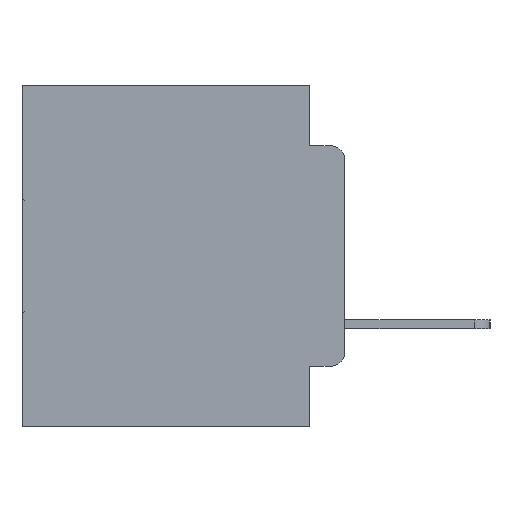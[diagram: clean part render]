
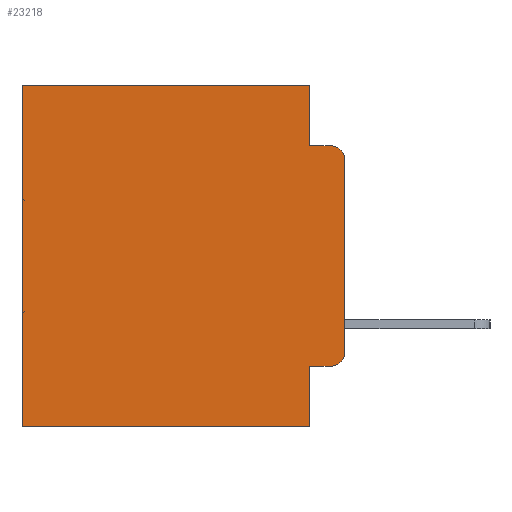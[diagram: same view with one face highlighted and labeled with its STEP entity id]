
A CAD part, left-side view. The second image highlights one B-rep face of the part: STEP entity #23218.
In plain terms, the highlighted planar face has unit normal (-1, 0, 0).
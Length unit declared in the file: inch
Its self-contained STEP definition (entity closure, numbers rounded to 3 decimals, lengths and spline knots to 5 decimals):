
#215 = DIRECTION ( 'NONE',  ( 0., 0., -1. ) ) ;
#223 = LINE ( 'NONE', #2752, #25096 ) ;
#811 = EDGE_CURVE ( 'NONE', #27575, #18160, #24040, .T. ) ;
#1923 = EDGE_CURVE ( 'NONE', #21573, #21307, #223, .T. ) ;
#2181 = CARTESIAN_POINT ( 'NONE',  ( 0.298, 0., 0. ) ) ;
#2608 = EDGE_CURVE ( 'NONE', #27176, #14300, #9049, .T. ) ;
#2657 = CARTESIAN_POINT ( 'NONE',  ( 0.298, 0., -0.5 ) ) ;
#2752 = CARTESIAN_POINT ( 'NONE',  ( 0.298, 0.051, -0.0885 ) ) ;
#2983 = CARTESIAN_POINT ( 'NONE',  ( 0.298, 0.02, -0.4115 ) ) ;
#3525 = EDGE_LOOP ( 'NONE', ( #14341, #7634, #15775, #22867, #12550, #25723, #14309, #5526, #22496, #13856 ) ) ;
#4274 = CARTESIAN_POINT ( 'NONE',  ( 0.298, 0.02, -0.3915 ) ) ;
#4275 = LINE ( 'NONE', #25701, #15556 ) ;
#4698 = DIRECTION ( 'NONE',  ( -1., 0., 0. ) ) ;
#5526 = ORIENTED_EDGE ( 'NONE', *, *, #7463, .F. ) ;
#6315 = VERTEX_POINT ( 'NONE', #19563 ) ;
#6690 = DIRECTION ( 'NONE',  ( 0., 0., -1. ) ) ;
#7463 = EDGE_CURVE ( 'NONE', #27575, #27176, #10236, .T. ) ;
#7634 = ORIENTED_EDGE ( 'NONE', *, *, #8484, .T. ) ;
#7880 = CIRCLE ( 'NONE', #20224, 0.02 ) ;
#8484 = EDGE_CURVE ( 'NONE', #24120, #21307, #11255, .T. ) ;
#9049 = LINE ( 'NONE', #2657, #14660 ) ;
#9115 = DIRECTION ( 'NONE',  ( 0., 0., -1. ) ) ;
#9828 = CARTESIAN_POINT ( 'NONE',  ( 0.298, 0., 0. ) ) ;
#9999 = DIRECTION ( 'NONE',  ( 0., 1., 0. ) ) ;
#10236 = LINE ( 'NONE', #17215, #22881 ) ;
#10637 = VECTOR ( 'NONE', #28673, 39.37008 ) ;
#10702 = CARTESIAN_POINT ( 'NONE',  ( 0.298, 0., -0.1085 ) ) ;
#10851 = VECTOR ( 'NONE', #9999, 39.37008 ) ;
#11255 = CIRCLE ( 'NONE', #20535, 0.02 ) ;
#11478 = DIRECTION ( 'NONE',  ( 0., 0., -1. ) ) ;
#11507 = CARTESIAN_POINT ( 'NONE',  ( 0.298, 0.473, 0. ) ) ;
#12235 = DIRECTION ( 'NONE',  ( 0., 0., -1. ) ) ;
#12550 = ORIENTED_EDGE ( 'NONE', *, *, #15513, .T. ) ;
#13628 = CARTESIAN_POINT ( 'NONE',  ( 0.298, 0.02, -0.0885 ) ) ;
#13856 = ORIENTED_EDGE ( 'NONE', *, *, #22452, .T. ) ;
#14300 = VERTEX_POINT ( 'NONE', #23668 ) ;
#14309 = ORIENTED_EDGE ( 'NONE', *, *, #2608, .F. ) ;
#14341 = ORIENTED_EDGE ( 'NONE', *, *, #24451, .F. ) ;
#14660 = VECTOR ( 'NONE', #19442, 39.37008 ) ;
#15508 = VECTOR ( 'NONE', #9115, 39.37008 ) ;
#15513 = EDGE_CURVE ( 'NONE', #6315, #24942, #17223, .T. ) ;
#15556 = VECTOR ( 'NONE', #11478, 39.37008 ) ;
#15655 = FACE_OUTER_BOUND ( 'NONE', #3525, .T. ) ;
#15775 = ORIENTED_EDGE ( 'NONE', *, *, #1923, .F. ) ;
#16238 = LINE ( 'NONE', #11507, #15508 ) ;
#16862 = AXIS2_PLACEMENT_3D ( 'NONE', #9828, #26424, #12235 ) ;
#17067 = CARTESIAN_POINT ( 'NONE',  ( 0.298, 0.051, -0.0885 ) ) ;
#17215 = CARTESIAN_POINT ( 'NONE',  ( 0.298, 0.051, 0. ) ) ;
#17223 = LINE ( 'NONE', #24221, #10851 ) ;
#18160 = VERTEX_POINT ( 'NONE', #2983 ) ;
#19022 = CARTESIAN_POINT ( 'NONE',  ( 0.298, 0.02, -0.1085 ) ) ;
#19291 = VECTOR ( 'NONE', #28391, 39.37008 ) ;
#19442 = DIRECTION ( 'NONE',  ( 0., 1., 0. ) ) ;
#19563 = CARTESIAN_POINT ( 'NONE',  ( 0.298, 0.051, 0. ) ) ;
#20224 = AXIS2_PLACEMENT_3D ( 'NONE', #4274, #20999, #6690 ) ;
#20280 = CARTESIAN_POINT ( 'NONE',  ( 0.298, 0.051, -0.5 ) ) ;
#20535 = AXIS2_PLACEMENT_3D ( 'NONE', #19022, #4698, #21439 ) ;
#20999 = DIRECTION ( 'NONE',  ( -1., 0., 0. ) ) ;
#21307 = VERTEX_POINT ( 'NONE', #13628 ) ;
#21439 = DIRECTION ( 'NONE',  ( 0., 0., -1. ) ) ;
#21573 = VERTEX_POINT ( 'NONE', #17067 ) ;
#21703 = PLANE ( 'NONE',  #16862 ) ;
#21880 = EDGE_CURVE ( 'NONE', #24942, #14300, #16238, .T. ) ;
#22452 = EDGE_CURVE ( 'NONE', #18160, #25117, #7880, .T. ) ;
#22496 = ORIENTED_EDGE ( 'NONE', *, *, #811, .T. ) ;
#22867 = ORIENTED_EDGE ( 'NONE', *, *, #25003, .F. ) ;
#22881 = VECTOR ( 'NONE', #215, 39.37008 ) ;
#23218 = ADVANCED_FACE ( 'NONE', ( #15655 ), #21703, .F. ) ;
#23668 = CARTESIAN_POINT ( 'NONE',  ( 0.298, 0.473, -0.5 ) ) ;
#23875 = CARTESIAN_POINT ( 'NONE',  ( 0.298, 0.051, -0.4115 ) ) ;
#24040 = LINE ( 'NONE', #28566, #10637 ) ;
#24120 = VERTEX_POINT ( 'NONE', #10702 ) ;
#24221 = CARTESIAN_POINT ( 'NONE',  ( 0.298, 0., 0. ) ) ;
#24451 = EDGE_CURVE ( 'NONE', #24120, #25117, #26312, .T. ) ;
#24942 = VERTEX_POINT ( 'NONE', #27742 ) ;
#25003 = EDGE_CURVE ( 'NONE', #6315, #21573, #4275, .T. ) ;
#25096 = VECTOR ( 'NONE', #28912, 39.37008 ) ;
#25117 = VERTEX_POINT ( 'NONE', #28525 ) ;
#25701 = CARTESIAN_POINT ( 'NONE',  ( 0.298, 0.051, 0. ) ) ;
#25723 = ORIENTED_EDGE ( 'NONE', *, *, #21880, .T. ) ;
#26312 = LINE ( 'NONE', #2181, #19291 ) ;
#26424 = DIRECTION ( 'NONE',  ( 1., 0., 0. ) ) ;
#27176 = VERTEX_POINT ( 'NONE', #20280 ) ;
#27575 = VERTEX_POINT ( 'NONE', #23875 ) ;
#27742 = CARTESIAN_POINT ( 'NONE',  ( 0.298, 0.473, 0. ) ) ;
#28391 = DIRECTION ( 'NONE',  ( 0., 0., -1. ) ) ;
#28525 = CARTESIAN_POINT ( 'NONE',  ( 0.298, 0., -0.3915 ) ) ;
#28566 = CARTESIAN_POINT ( 'NONE',  ( 0.298, 0.051, -0.4115 ) ) ;
#28673 = DIRECTION ( 'NONE',  ( 0., -1., 0. ) ) ;
#28912 = DIRECTION ( 'NONE',  ( 0., -1., 0. ) ) ;
